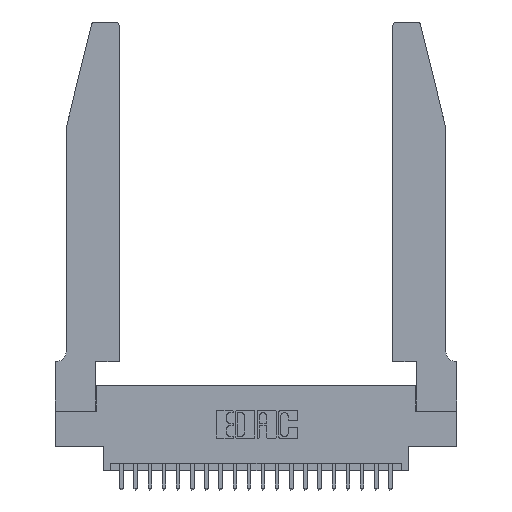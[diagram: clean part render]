
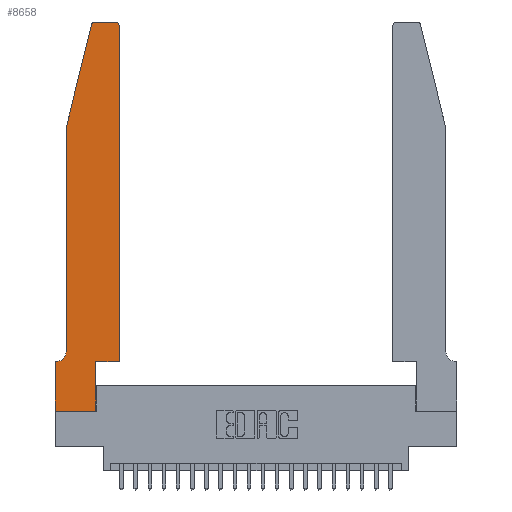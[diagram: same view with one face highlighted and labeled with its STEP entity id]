
A CAD part, top view. The second image highlights one B-rep face of the part: STEP entity #8658.
In plain terms, the highlighted planar face has unit normal (0, 0, 1).
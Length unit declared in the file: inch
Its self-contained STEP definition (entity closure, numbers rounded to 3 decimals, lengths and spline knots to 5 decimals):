
#22 = LINE ( 'NONE', #5645, #18378 ) ;
#873 = CARTESIAN_POINT ( 'NONE',  ( 0.0055, 0.35, 0.37 ) ) ;
#966 = EDGE_CURVE ( 'NONE', #7930, #14631, #16616, .T. ) ;
#1345 = DIRECTION ( 'NONE',  ( 1., 0., 0. ) ) ;
#1904 = DIRECTION ( 'NONE',  ( 0., -1., 0. ) ) ;
#2078 = EDGE_CURVE ( 'NONE', #19141, #8566, #14879, .T. ) ;
#2085 = VERTEX_POINT ( 'NONE', #9343 ) ;
#2210 = AXIS2_PLACEMENT_3D ( 'NONE', #19806, #9042, #21597 ) ;
#2666 = CARTESIAN_POINT ( 'NONE',  ( 0.0755, 0.42, 0.37 ) ) ;
#2846 = AXIS2_PLACEMENT_3D ( 'NONE', #4213, #7927, #20521 ) ;
#3053 = ORIENTED_EDGE ( 'NONE', *, *, #17065, .T. ) ;
#3270 = ORIENTED_EDGE ( 'NONE', *, *, #6920, .T. ) ;
#3505 = CIRCLE ( 'NONE', #2210, 0.07 ) ;
#3862 = EDGE_LOOP ( 'NONE', ( #4361, #18128, #4689, #22461, #19251, #15873, #7686, #3270, #16223, #9775, #3053, #22997 ) ) ;
#4213 = CARTESIAN_POINT ( 'NONE',  ( 0., 0.35, 0.37 ) ) ;
#4361 = ORIENTED_EDGE ( 'NONE', *, *, #966, .T. ) ;
#4689 = ORIENTED_EDGE ( 'NONE', *, *, #15105, .T. ) ;
#5201 = CARTESIAN_POINT ( 'NONE',  ( 0.2605, 2.75, 0.37 ) ) ;
#5553 = AXIS2_PLACEMENT_3D ( 'NONE', #16463, #5608, #18283 ) ;
#5608 = DIRECTION ( 'NONE',  ( 0., 0., 1. ) ) ;
#5645 = CARTESIAN_POINT ( 'NONE',  ( 0.4505, 0.35, 0.37 ) ) ;
#6211 = DIRECTION ( 'NONE',  ( -1., 0., 0. ) ) ;
#6269 = LINE ( 'NONE', #13145, #11132 ) ;
#6482 = CIRCLE ( 'NONE', #21126, 0.03 ) ;
#6920 = EDGE_CURVE ( 'NONE', #2085, #19141, #8442, .T. ) ;
#7088 = VECTOR ( 'NONE', #10906, 39.37008 ) ;
#7090 = EDGE_CURVE ( 'NONE', #17343, #2085, #19424, .T. ) ;
#7152 = VERTEX_POINT ( 'NONE', #15034 ) ;
#7394 = CARTESIAN_POINT ( 'NONE',  ( 0.4205, 2.75, 0.37 ) ) ;
#7494 = DIRECTION ( 'NONE',  ( 0., 1., 0. ) ) ;
#7567 = VECTOR ( 'NONE', #13330, 39.37008 ) ;
#7679 = CARTESIAN_POINT ( 'NONE',  ( 0., 0., 0.37 ) ) ;
#7686 = ORIENTED_EDGE ( 'NONE', *, *, #7090, .T. ) ;
#7927 = DIRECTION ( 'NONE',  ( 0., 0., 1. ) ) ;
#7930 = VERTEX_POINT ( 'NONE', #7394 ) ;
#8430 = CARTESIAN_POINT ( 'NONE',  ( 0.0755, 2., 0.37 ) ) ;
#8442 = LINE ( 'NONE', #17940, #17455 ) ;
#8504 = CARTESIAN_POINT ( 'NONE',  ( 0.2865, 0., 0.37 ) ) ;
#8566 = VERTEX_POINT ( 'NONE', #11345 ) ;
#8658 = ADVANCED_FACE ( 'NONE', ( #23536 ), #13307, .T. ) ;
#8792 = VECTOR ( 'NONE', #12061, 39.37008 ) ;
#8990 = CARTESIAN_POINT ( 'NONE',  ( 0.4505, 0.35, 0.37 ) ) ;
#9042 = DIRECTION ( 'NONE',  ( 0., 0., -1. ) ) ;
#9343 = CARTESIAN_POINT ( 'NONE',  ( 0., 0., 0.37 ) ) ;
#9411 = VERTEX_POINT ( 'NONE', #873 ) ;
#9775 = ORIENTED_EDGE ( 'NONE', *, *, #11124, .T. ) ;
#10435 = EDGE_CURVE ( 'NONE', #20763, #7930, #18733, .T. ) ;
#10906 = DIRECTION ( 'NONE',  ( 1., 0., 0. ) ) ;
#11124 = EDGE_CURVE ( 'NONE', #8566, #11711, #21463, .T. ) ;
#11132 = VECTOR ( 'NONE', #14958, 39.37008 ) ;
#11345 = CARTESIAN_POINT ( 'NONE',  ( 0.2865, 0.35, 0.37 ) ) ;
#11509 = EDGE_CURVE ( 'NONE', #18899, #17371, #18401, .T. ) ;
#11625 = EDGE_CURVE ( 'NONE', #14631, #7152, #6482, .T. ) ;
#11711 = VERTEX_POINT ( 'NONE', #8990 ) ;
#11926 = CARTESIAN_POINT ( 'NONE',  ( 0.0755, 0.35, 0.37 ) ) ;
#12061 = DIRECTION ( 'NONE',  ( 0., -1., 0. ) ) ;
#12377 = DIRECTION ( 'NONE',  ( 0., 0., 1. ) ) ;
#12395 = CARTESIAN_POINT ( 'NONE',  ( 0.0755, 2., 0.37 ) ) ;
#13145 = CARTESIAN_POINT ( 'NONE',  ( 0.0755, 2., 0.37 ) ) ;
#13307 = PLANE ( 'NONE',  #2846 ) ;
#13330 = DIRECTION ( 'NONE',  ( -1., 0., 0. ) ) ;
#13568 = CARTESIAN_POINT ( 'NONE',  ( 0., 0.35, 0.37 ) ) ;
#14631 = VERTEX_POINT ( 'NONE', #20835 ) ;
#14879 = LINE ( 'NONE', #16505, #19069 ) ;
#14958 = DIRECTION ( 'NONE',  ( -0.239, -0.971, 0. ) ) ;
#15034 = CARTESIAN_POINT ( 'NONE',  ( 0.25487, 2.72718, 0.37 ) ) ;
#15105 = EDGE_CURVE ( 'NONE', #7152, #18899, #6269, .T. ) ;
#15873 = ORIENTED_EDGE ( 'NONE', *, *, #16719, .T. ) ;
#16117 = LINE ( 'NONE', #11926, #22000 ) ;
#16223 = ORIENTED_EDGE ( 'NONE', *, *, #2078, .T. ) ;
#16463 = CARTESIAN_POINT ( 'NONE',  ( 0.4205, 2.72, 0.37 ) ) ;
#16505 = CARTESIAN_POINT ( 'NONE',  ( 0.2865, 0.35, 0.37 ) ) ;
#16616 = LINE ( 'NONE', #5201, #7567 ) ;
#16719 = EDGE_CURVE ( 'NONE', #9411, #17343, #16117, .T. ) ;
#17065 = EDGE_CURVE ( 'NONE', #11711, #20763, #22, .T. ) ;
#17343 = VERTEX_POINT ( 'NONE', #13568 ) ;
#17371 = VERTEX_POINT ( 'NONE', #2666 ) ;
#17455 = VECTOR ( 'NONE', #21526, 39.37008 ) ;
#17940 = CARTESIAN_POINT ( 'NONE',  ( 0., 0., 0.37 ) ) ;
#18128 = ORIENTED_EDGE ( 'NONE', *, *, #11625, .T. ) ;
#18283 = DIRECTION ( 'NONE',  ( 1., 0., 0. ) ) ;
#18297 = EDGE_CURVE ( 'NONE', #17371, #9411, #3505, .T. ) ;
#18322 = DIRECTION ( 'NONE',  ( 0., 1., 0. ) ) ;
#18378 = VECTOR ( 'NONE', #18322, 39.37008 ) ;
#18401 = LINE ( 'NONE', #8430, #8792 ) ;
#18733 = CIRCLE ( 'NONE', #5553, 0.03 ) ;
#18876 = VECTOR ( 'NONE', #1904, 39.37008 ) ;
#18899 = VERTEX_POINT ( 'NONE', #12395 ) ;
#19069 = VECTOR ( 'NONE', #7494, 39.37008 ) ;
#19141 = VERTEX_POINT ( 'NONE', #8504 ) ;
#19251 = ORIENTED_EDGE ( 'NONE', *, *, #18297, .T. ) ;
#19424 = LINE ( 'NONE', #7679, #18876 ) ;
#19806 = CARTESIAN_POINT ( 'NONE',  ( 0.0055, 0.42, 0.37 ) ) ;
#20521 = DIRECTION ( 'NONE',  ( 1., 0., 0. ) ) ;
#20763 = VERTEX_POINT ( 'NONE', #22700 ) ;
#20835 = CARTESIAN_POINT ( 'NONE',  ( 0.284, 2.75, 0.37 ) ) ;
#21126 = AXIS2_PLACEMENT_3D ( 'NONE', #23088, #12377, #1345 ) ;
#21463 = LINE ( 'NONE', #21653, #7088 ) ;
#21526 = DIRECTION ( 'NONE',  ( 1., 0., 0. ) ) ;
#21597 = DIRECTION ( 'NONE',  ( -1., 0., 0. ) ) ;
#21653 = CARTESIAN_POINT ( 'NONE',  ( 0.4505, 0.35, 0.37 ) ) ;
#22000 = VECTOR ( 'NONE', #6211, 39.37008 ) ;
#22461 = ORIENTED_EDGE ( 'NONE', *, *, #11509, .T. ) ;
#22700 = CARTESIAN_POINT ( 'NONE',  ( 0.4505, 2.72, 0.37 ) ) ;
#22997 = ORIENTED_EDGE ( 'NONE', *, *, #10435, .T. ) ;
#23088 = CARTESIAN_POINT ( 'NONE',  ( 0.284, 2.72, 0.37 ) ) ;
#23536 = FACE_OUTER_BOUND ( 'NONE', #3862, .T. ) ;
